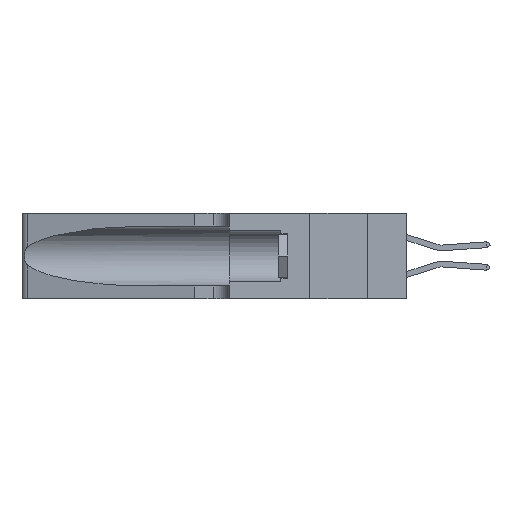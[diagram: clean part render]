
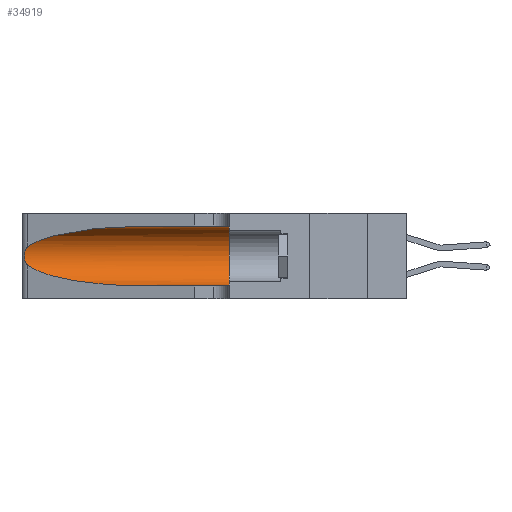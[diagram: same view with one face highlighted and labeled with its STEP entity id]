
A CAD part, left-side view. The second image highlights one B-rep face of the part: STEP entity #34919.
In plain terms, the highlighted cylindrical face has radius 3.308 mm (diameter 6.617 mm), a partial arc.
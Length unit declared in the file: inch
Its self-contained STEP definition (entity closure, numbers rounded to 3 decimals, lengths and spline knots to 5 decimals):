
#430 = CARTESIAN_POINT ( 'NONE',  ( 0.25854, 1.2359, 0.20912 ) ) ;
#709 = VERTEX_POINT ( 'NONE', #3810 ) ;
#992 = LINE ( 'NONE', #6687, #7682 ) ;
#1083 = CARTESIAN_POINT ( 'NONE',  ( 0.25487, 1.22718, 0.14631 ) ) ;
#1850 = CARTESIAN_POINT ( 'NONE',  ( 0.1305, 0.72297, 0.31525 ) ) ;
#2896 = DIRECTION ( 'NONE',  ( 0., -1., 0. ) ) ;
#3201 = CARTESIAN_POINT ( 'NONE',  ( 0.25555, 1.22994, 0.2215 ) ) ;
#3322 = CARTESIAN_POINT ( 'NONE',  ( 0.26075, 1.23896, 0.19203 ) ) ;
#3686 = VERTEX_POINT ( 'NONE', #9156 ) ;
#3810 = CARTESIAN_POINT ( 'NONE',  ( 0.1305, 0.35, 0.05475 ) ) ;
#4523 = FACE_OUTER_BOUND ( 'NONE', #23349, .T. ) ;
#4739 = CARTESIAN_POINT ( 'NONE',  ( 0.1305, 0.35, 0.31525 ) ) ;
#5297 = CIRCLE ( 'NONE', #30365, 0.13025 ) ;
#5770 = CARTESIAN_POINT ( 'NONE',  ( 0.1305, 1.61858, 0.31525 ) ) ;
#6187 = CARTESIAN_POINT ( 'NONE',  ( 0.26017, 1.23833, 0.17102 ) ) ;
#6687 = CARTESIAN_POINT ( 'NONE',  ( 0.1305, 1.61858, 0.05475 ) ) ;
#6818 = CARTESIAN_POINT ( 'NONE',  ( 0.18966, 0.96281, 0.05475 ) ) ;
#6971 = VECTOR ( 'NONE', #2896, 39.37008 ) ;
#7682 = VECTOR ( 'NONE', #34387, 39.37008 ) ;
#7861 = LINE ( 'NONE', #5770, #6971 ) ;
#8975 = CARTESIAN_POINT ( 'NONE',  ( 0.25789, 1.23486, 0.15765 ) ) ;
#9156 = CARTESIAN_POINT ( 'NONE',  ( 0.1305, 0.72297, 0.05475 ) ) ;
#9717 = VERTEX_POINT ( 'NONE', #11461 ) ;
#10168 = CYLINDRICAL_SURFACE ( 'NONE', #35729, 0.13025 ) ;
#10237 = CARTESIAN_POINT ( 'NONE',  ( 0.1305, 0.35, 0.185 ) ) ;
#11461 = CARTESIAN_POINT ( 'NONE',  ( 0.1305, 0.72297, 0.31525 ) ) ;
#11789 = CARTESIAN_POINT ( 'NONE',  ( 0.25555, 1.22993, 0.14849 ) ) ;
#13054 = DIRECTION ( 'NONE',  ( 0., 0., 1. ) ) ;
#13284 = CARTESIAN_POINT ( 'NONE',  ( 0.2373, 1.15595, 0.28018 ) ) ;
#13389 = VERTEX_POINT ( 'NONE', #19737 ) ;
#13653 = ORIENTED_EDGE ( 'NONE', *, *, #23202, .T. ) ;
#13999 = ORIENTED_EDGE ( 'NONE', *, *, #28352, .F. ) ;
#14589 = VERTEX_POINT ( 'NONE', #4739 ) ;
#15133 = CARTESIAN_POINT ( 'NONE',  ( 0.2373, 1.15595, 0.08982 ) ) ;
#15999 = CARTESIAN_POINT ( 'NONE',  ( 0.18966, 0.96281, 0.31525 ) ) ;
#16209 =( BOUNDED_CURVE ( )  B_SPLINE_CURVE ( 3, ( #1850, #15999, #13284, #32593 ),
 .UNSPECIFIED., .F., .T. ) 
 B_SPLINE_CURVE_WITH_KNOTS ( ( 4, 4 ),
 ( 1.5708, 2.84003 ),
 .UNSPECIFIED. ) 
 CURVE ( )  GEOMETRIC_REPRESENTATION_ITEM ( )  RATIONAL_B_SPLINE_CURVE ( ( 1., 0.87, 0.87, 1. ) ) 
 REPRESENTATION_ITEM ( '' )  );
#17298 = CARTESIAN_POINT ( 'NONE',  ( 0.25787, 1.23484, 0.2124 ) ) ;
#17940 = ORIENTED_EDGE ( 'NONE', *, *, #29058, .T. ) ;
#19468 = DIRECTION ( 'NONE',  ( 0., -1., 0. ) ) ;
#19737 = CARTESIAN_POINT ( 'NONE',  ( 0.25487, 1.22718, 0.14631 ) ) ;
#19908 = ORIENTED_EDGE ( 'NONE', *, *, #20064, .T. ) ;
#20061 = EDGE_CURVE ( 'NONE', #3686, #709, #992, .T. ) ;
#20064 = EDGE_CURVE ( 'NONE', #13389, #3686, #22665, .T. ) ;
#20080 = CARTESIAN_POINT ( 'NONE',  ( 0.26018, 1.23835, 0.19895 ) ) ;
#22665 =( BOUNDED_CURVE ( )  B_SPLINE_CURVE ( 3, ( #1083, #15133, #6818, #26282 ),
 .UNSPECIFIED., .F., .F. ) 
 B_SPLINE_CURVE_WITH_KNOTS ( ( 4, 4 ),
 ( 3.44316, 4.71239 ),
 .UNSPECIFIED. ) 
 CURVE ( )  GEOMETRIC_REPRESENTATION_ITEM ( )  RATIONAL_B_SPLINE_CURVE ( ( 1., 0.87, 0.87, 1. ) ) 
 REPRESENTATION_ITEM ( '' )  );
#22886 = CARTESIAN_POINT ( 'NONE',  ( 0.26075, 1.23896, 0.178 ) ) ;
#23202 = EDGE_CURVE ( 'NONE', #9717, #27259, #16209, .T. ) ;
#23349 = EDGE_LOOP ( 'NONE', ( #13653, #17940, #19908, #27527, #28954, #13999 ) ) ;
#23685 = EDGE_CURVE ( 'NONE', #14589, #709, #5297, .T. ) ;
#25649 = CARTESIAN_POINT ( 'NONE',  ( 0.25856, 1.23593, 0.16098 ) ) ;
#26282 = CARTESIAN_POINT ( 'NONE',  ( 0.1305, 0.72297, 0.05475 ) ) ;
#26406 = B_SPLINE_CURVE_WITH_KNOTS ( 'NONE', 3,
 ( #31013, #3201, #33758, #17298, #430, #20080, #3322, #22886, #6187, #25649, #8975, #28400, #11789, #31130 ),
 .UNSPECIFIED., .F., .F.,
 ( 4, 2, 2, 2, 2, 2, 4 ),
 ( 0., 0.00027, 0.00053, 0.00107, 0.0016, 0.00187, 0.00214 ),
 .UNSPECIFIED. ) ;
#27259 = VERTEX_POINT ( 'NONE', #34591 ) ;
#27527 = ORIENTED_EDGE ( 'NONE', *, *, #20061, .T. ) ;
#27689 = CARTESIAN_POINT ( 'NONE',  ( 0.1305, 1.61858, 0.185 ) ) ;
#28352 = EDGE_CURVE ( 'NONE', #9717, #14589, #7861, .T. ) ;
#28400 = CARTESIAN_POINT ( 'NONE',  ( 0.25639, 1.23186, 0.15144 ) ) ;
#28954 = ORIENTED_EDGE ( 'NONE', *, *, #23685, .F. ) ;
#29058 = EDGE_CURVE ( 'NONE', #27259, #13389, #26406, .T. ) ;
#29633 = DIRECTION ( 'NONE',  ( 0., 1., 0. ) ) ;
#30365 = AXIS2_PLACEMENT_3D ( 'NONE', #10237, #29633, #13054 ) ;
#31013 = CARTESIAN_POINT ( 'NONE',  ( 0.25487, 1.22718, 0.22369 ) ) ;
#31130 = CARTESIAN_POINT ( 'NONE',  ( 0.25487, 1.22718, 0.14631 ) ) ;
#32593 = CARTESIAN_POINT ( 'NONE',  ( 0.25487, 1.22718, 0.22369 ) ) ;
#33163 = DIRECTION ( 'NONE',  ( 0., 0., -1. ) ) ;
#33758 = CARTESIAN_POINT ( 'NONE',  ( 0.25639, 1.23184, 0.21858 ) ) ;
#34387 = DIRECTION ( 'NONE',  ( 0., -1., 0. ) ) ;
#34591 = CARTESIAN_POINT ( 'NONE',  ( 0.25487, 1.22718, 0.22369 ) ) ;
#34919 = ADVANCED_FACE ( 'NONE', ( #4523 ), #10168, .F. ) ;
#35729 = AXIS2_PLACEMENT_3D ( 'NONE', #27689, #19468, #33163 ) ;
